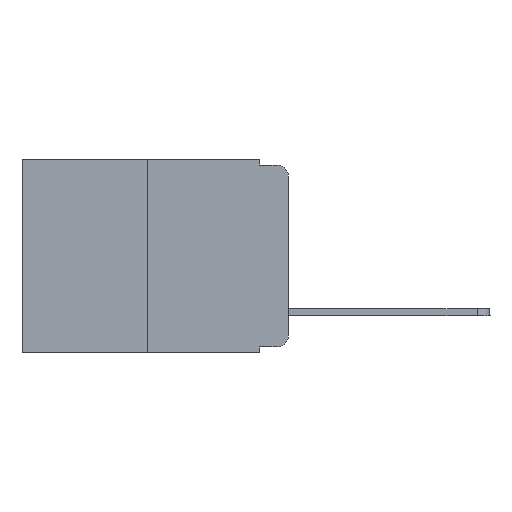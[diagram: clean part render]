
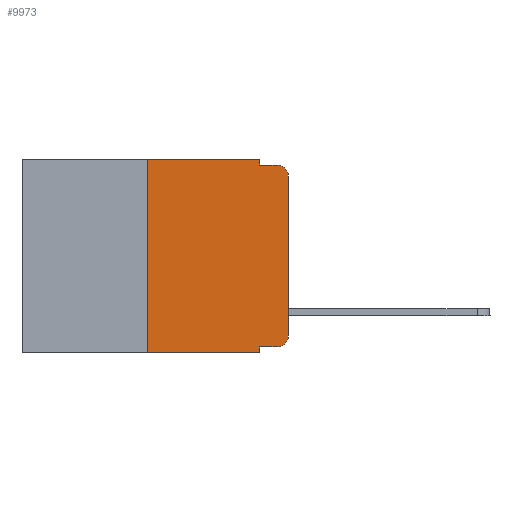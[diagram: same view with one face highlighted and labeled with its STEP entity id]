
A CAD part, left-side view. The second image highlights one B-rep face of the part: STEP entity #9973.
In plain terms, the highlighted planar face has unit normal (-1, 0, 0).
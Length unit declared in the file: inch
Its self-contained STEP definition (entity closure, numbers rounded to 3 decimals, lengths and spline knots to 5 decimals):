
#326 = LINE ( 'NONE', #13288, #2699 ) ;
#530 = EDGE_CURVE ( 'NONE', #6710, #10018, #326, .T. ) ;
#1013 = VECTOR ( 'NONE', #13830, 39.37008 ) ;
#1097 = CARTESIAN_POINT ( 'NONE',  ( 0., 0.02, -0.333 ) ) ;
#1115 = CARTESIAN_POINT ( 'NONE',  ( 0., 0.051, 0. ) ) ;
#1144 = VECTOR ( 'NONE', #13415, 39.37008 ) ;
#1220 = CARTESIAN_POINT ( 'NONE',  ( 0., 0.473, -0.343 ) ) ;
#1287 = EDGE_CURVE ( 'NONE', #3040, #14666, #14157, .T. ) ;
#1295 = CARTESIAN_POINT ( 'NONE',  ( 0., 0.25, 0. ) ) ;
#1370 = EDGE_CURVE ( 'NONE', #2844, #3747, #2461, .T. ) ;
#1633 = ORIENTED_EDGE ( 'NONE', *, *, #4634, .T. ) ;
#2222 = VECTOR ( 'NONE', #11017, 39.37008 ) ;
#2461 = LINE ( 'NONE', #11067, #14357 ) ;
#2699 = VECTOR ( 'NONE', #13236, 39.37008 ) ;
#2844 = VERTEX_POINT ( 'NONE', #6349 ) ;
#2931 = AXIS2_PLACEMENT_3D ( 'NONE', #13949, #7770, #6906 ) ;
#2986 = DIRECTION ( 'NONE',  ( -1., 0., 0. ) ) ;
#3040 = VERTEX_POINT ( 'NONE', #7023 ) ;
#3223 = LINE ( 'NONE', #1115, #10242 ) ;
#3747 = VERTEX_POINT ( 'NONE', #6720 ) ;
#3806 = DIRECTION ( 'NONE',  ( 0., 0., 1. ) ) ;
#3814 = FACE_OUTER_BOUND ( 'NONE', #14850, .T. ) ;
#4137 = CARTESIAN_POINT ( 'NONE',  ( 0., 0.25, 0. ) ) ;
#4182 = LINE ( 'NONE', #10914, #2222 ) ;
#4219 = DIRECTION ( 'NONE',  ( 0., 0., -1. ) ) ;
#4555 = ORIENTED_EDGE ( 'NONE', *, *, #7592, .T. ) ;
#4634 = EDGE_CURVE ( 'NONE', #6710, #12392, #4182, .T. ) ;
#5071 = AXIS2_PLACEMENT_3D ( 'NONE', #7682, #8870, #8926 ) ;
#5489 = CIRCLE ( 'NONE', #13005, 0.02 ) ;
#6143 = DIRECTION ( 'NONE',  ( 0., -1., 0. ) ) ;
#6258 = EDGE_CURVE ( 'NONE', #10544, #9786, #13689, .T. ) ;
#6279 = ORIENTED_EDGE ( 'NONE', *, *, #1370, .T. ) ;
#6313 = DIRECTION ( 'NONE',  ( 0., 0., -1. ) ) ;
#6349 = CARTESIAN_POINT ( 'NONE',  ( 0., 0., -0.313 ) ) ;
#6549 = CARTESIAN_POINT ( 'NONE',  ( 0., 0.051, 0. ) ) ;
#6710 = VERTEX_POINT ( 'NONE', #15176 ) ;
#6720 = CARTESIAN_POINT ( 'NONE',  ( 0., 0., -0.03 ) ) ;
#6877 = DIRECTION ( 'NONE',  ( 0., -1., 0. ) ) ;
#6906 = DIRECTION ( 'NONE',  ( 0., 0., -1. ) ) ;
#7023 = CARTESIAN_POINT ( 'NONE',  ( 0., 0.051, -0.01 ) ) ;
#7372 = EDGE_CURVE ( 'NONE', #10544, #10018, #11127, .T. ) ;
#7592 = EDGE_CURVE ( 'NONE', #3747, #14666, #5489, .T. ) ;
#7682 = CARTESIAN_POINT ( 'NONE',  ( 0., 0.02, -0.313 ) ) ;
#7770 = DIRECTION ( 'NONE',  ( 1., 0., 0. ) ) ;
#7854 = EDGE_CURVE ( 'NONE', #9786, #9608, #16151, .T. ) ;
#7857 = ORIENTED_EDGE ( 'NONE', *, *, #7854, .F. ) ;
#8010 = EDGE_CURVE ( 'NONE', #12392, #2844, #10340, .T. ) ;
#8474 = ORIENTED_EDGE ( 'NONE', *, *, #1287, .F. ) ;
#8870 = DIRECTION ( 'NONE',  ( -1., 0., 0. ) ) ;
#8893 = ORIENTED_EDGE ( 'NONE', *, *, #530, .F. ) ;
#8926 = DIRECTION ( 'NONE',  ( 0., 0., -1. ) ) ;
#8965 = PLANE ( 'NONE',  #2931 ) ;
#9093 = ORIENTED_EDGE ( 'NONE', *, *, #8010, .T. ) ;
#9332 = CARTESIAN_POINT ( 'NONE',  ( 0., 0.051, -0.01 ) ) ;
#9608 = VERTEX_POINT ( 'NONE', #6549 ) ;
#9786 = VERTEX_POINT ( 'NONE', #4137 ) ;
#9973 = ADVANCED_FACE ( 'NONE', ( #3814 ), #8965, .F. ) ;
#10018 = VERTEX_POINT ( 'NONE', #14336 ) ;
#10242 = VECTOR ( 'NONE', #6313, 39.37008 ) ;
#10340 = CIRCLE ( 'NONE', #5071, 0.02 ) ;
#10464 = CARTESIAN_POINT ( 'NONE',  ( 0., 0.02, -0.03 ) ) ;
#10544 = VERTEX_POINT ( 'NONE', #12573 ) ;
#10670 = CARTESIAN_POINT ( 'NONE',  ( 0., 0.02, -0.01 ) ) ;
#10914 = CARTESIAN_POINT ( 'NONE',  ( 0., 0.051, -0.333 ) ) ;
#11017 = DIRECTION ( 'NONE',  ( 0., -1., 0. ) ) ;
#11049 = CARTESIAN_POINT ( 'NONE',  ( 0., 0.473, 0. ) ) ;
#11067 = CARTESIAN_POINT ( 'NONE',  ( 0., 0., 0. ) ) ;
#11127 = LINE ( 'NONE', #1220, #14253 ) ;
#11784 = EDGE_CURVE ( 'NONE', #9608, #3040, #3223, .T. ) ;
#12392 = VERTEX_POINT ( 'NONE', #1097 ) ;
#12573 = CARTESIAN_POINT ( 'NONE',  ( 0., 0.25, -0.343 ) ) ;
#13005 = AXIS2_PLACEMENT_3D ( 'NONE', #10464, #2986, #4219 ) ;
#13236 = DIRECTION ( 'NONE',  ( 0., 0., -1. ) ) ;
#13288 = CARTESIAN_POINT ( 'NONE',  ( 0., 0.051, 0. ) ) ;
#13415 = DIRECTION ( 'NONE',  ( 0., -1., 0. ) ) ;
#13689 = LINE ( 'NONE', #1295, #1013 ) ;
#13745 = VECTOR ( 'NONE', #6877, 39.37008 ) ;
#13830 = DIRECTION ( 'NONE',  ( 0., 0., 1. ) ) ;
#13949 = CARTESIAN_POINT ( 'NONE',  ( 0., 0.473, 0. ) ) ;
#14122 = ORIENTED_EDGE ( 'NONE', *, *, #7372, .T. ) ;
#14157 = LINE ( 'NONE', #9332, #13745 ) ;
#14253 = VECTOR ( 'NONE', #6143, 39.37008 ) ;
#14336 = CARTESIAN_POINT ( 'NONE',  ( 0., 0.051, -0.343 ) ) ;
#14357 = VECTOR ( 'NONE', #3806, 39.37008 ) ;
#14459 = ORIENTED_EDGE ( 'NONE', *, *, #6258, .F. ) ;
#14666 = VERTEX_POINT ( 'NONE', #10670 ) ;
#14850 = EDGE_LOOP ( 'NONE', ( #6279, #4555, #8474, #15280, #7857, #14459, #14122, #8893, #1633, #9093 ) ) ;
#15176 = CARTESIAN_POINT ( 'NONE',  ( 0., 0.051, -0.333 ) ) ;
#15280 = ORIENTED_EDGE ( 'NONE', *, *, #11784, .F. ) ;
#16151 = LINE ( 'NONE', #11049, #1144 ) ;
